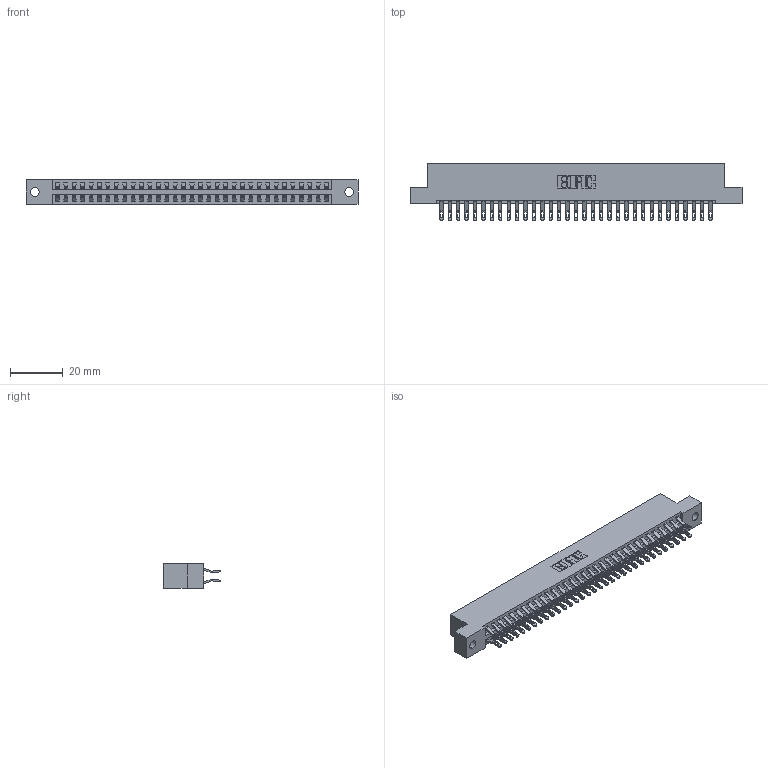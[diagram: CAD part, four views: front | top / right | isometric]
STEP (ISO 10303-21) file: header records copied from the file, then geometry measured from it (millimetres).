
FILE_DESCRIPTION (( 'STEP AP203' ), '1' );
FILE_NAME ('396-066-555-202.STEP', '2018-09-08T19:35:42', ( '' ), ( '' ), 'SwSTEP 2.0', 'SolidWorks 2016', '' );
FILE_SCHEMA (( 'CONFIG_CONTROL_DESIGN' ));
Length unit declared in the file: inch
Products named in the file (3): 396-066-555-202; 346 Part_Flush Mounting Lugs - 0.128 Dia; 345-292-001_555 Tail
Assembly tree (67 placements, depth 2):
  396-066-555-202
    346 Part_Flush Mounting Lugs - 0.128 Dia
    345-292-001_555 Tail  x66
Bounding box: 125.35 x 21.46 x 9.4 mm (x, y, z)
Volume: 11522.6 mm3; surface area: 17151.4 mm2
Topology: 1 solids, 67 shells, 3884 faces, 12407 edges, 8270 vertices
Faces by surface type: plane 2254, cylinder 1630
Entity records: 23077 total; most frequent: CARTESIAN_POINT 3850, ORIENTED_EDGE 3754, DIRECTION 3413, EDGE_CURVE 1877, VECTOR 1593, LINE 1593, VERTEX_POINT 1250, AXIS2_PLACEMENT_3D 910
